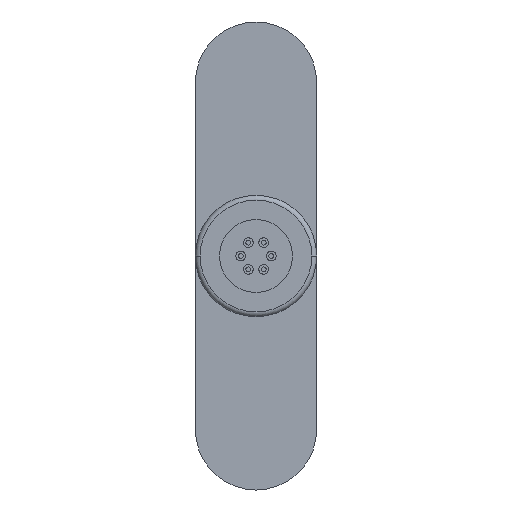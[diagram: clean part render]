
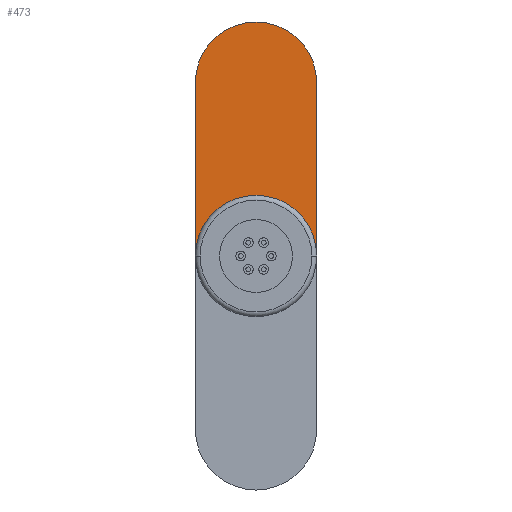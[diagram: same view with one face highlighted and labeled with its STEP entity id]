
A CAD part, left-side view. The second image highlights one B-rep face of the part: STEP entity #473.
In plain terms, the highlighted planar face has unit normal (-1, 0, 0).
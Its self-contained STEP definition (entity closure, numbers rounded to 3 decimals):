
#41 = CARTESIAN_POINT ( 'NONE',  ( 56.3, 0., 0. ) ) ;
#128 = ORIENTED_EDGE ( 'NONE', *, *, #1739, .T. ) ;
#296 = ORIENTED_EDGE ( 'NONE', *, *, #1488, .F. ) ;
#389 = DIRECTION ( 'NONE',  ( 1., 0., 0. ) ) ;
#422 = PLANE ( 'NONE',  #2279 ) ;
#450 = VERTEX_POINT ( 'NONE', #1172 ) ;
#473 = ADVANCED_FACE ( 'NONE', ( #2866 ), #422, .F. ) ;
#717 = DIRECTION ( 'NONE',  ( 0., -1., 0. ) ) ;
#743 = DIRECTION ( 'NONE',  ( 0., -1., 0. ) ) ;
#779 = DIRECTION ( 'NONE',  ( -1., 0., 0. ) ) ;
#783 = DIRECTION ( 'NONE',  ( 0., 0., -1. ) ) ;
#821 = EDGE_CURVE ( 'NONE', #450, #3025, #1712, .T. ) ;
#884 = VECTOR ( 'NONE', #2243, 1000. ) ;
#905 = LINE ( 'NONE', #2281, #884 ) ;
#1121 = CARTESIAN_POINT ( 'NONE',  ( 56.3, -3.75, 0. ) ) ;
#1144 = CARTESIAN_POINT ( 'NONE',  ( 56.3, 0., 0. ) ) ;
#1172 = CARTESIAN_POINT ( 'NONE',  ( 56.3, -3.75, 10.7 ) ) ;
#1200 = CARTESIAN_POINT ( 'NONE',  ( 56.3, 3.75, 0. ) ) ;
#1422 = CARTESIAN_POINT ( 'NONE',  ( 56.3, 0., 10.7 ) ) ;
#1429 = AXIS2_PLACEMENT_3D ( 'NONE', #1422, #779, #717 ) ;
#1488 = EDGE_CURVE ( 'NONE', #3967, #3025, #905, .T. ) ;
#1597 = CARTESIAN_POINT ( 'NONE',  ( 56.3, 3.75, 10.7 ) ) ;
#1712 = CIRCLE ( 'NONE', #1429, 3.75 ) ;
#1739 = EDGE_CURVE ( 'NONE', #3967, #3236, #3593, .T. ) ;
#2243 = DIRECTION ( 'NONE',  ( 0., 0., 1. ) ) ;
#2279 = AXIS2_PLACEMENT_3D ( 'NONE', #1144, #3131, #743 ) ;
#2281 = CARTESIAN_POINT ( 'NONE',  ( 56.3, 3.75, 14.45 ) ) ;
#2599 = ORIENTED_EDGE ( 'NONE', *, *, #3233, .F. ) ;
#2653 = VECTOR ( 'NONE', #783, 1000. ) ;
#2786 = DIRECTION ( 'NONE',  ( 0., -1., 0. ) ) ;
#2866 = FACE_OUTER_BOUND ( 'NONE', #3850, .T. ) ;
#3025 = VERTEX_POINT ( 'NONE', #1597 ) ;
#3131 = DIRECTION ( 'NONE',  ( 1., 0., 0. ) ) ;
#3233 = EDGE_CURVE ( 'NONE', #450, #3236, #3541, .T. ) ;
#3236 = VERTEX_POINT ( 'NONE', #1121 ) ;
#3541 = LINE ( 'NONE', #4187, #2653 ) ;
#3593 = CIRCLE ( 'NONE', #4025, 3.75 ) ;
#3835 = ORIENTED_EDGE ( 'NONE', *, *, #821, .T. ) ;
#3850 = EDGE_LOOP ( 'NONE', ( #296, #128, #2599, #3835 ) ) ;
#3967 = VERTEX_POINT ( 'NONE', #1200 ) ;
#4025 = AXIS2_PLACEMENT_3D ( 'NONE', #41, #389, #2786 ) ;
#4187 = CARTESIAN_POINT ( 'NONE',  ( 56.3, -3.75, 14.45 ) ) ;
